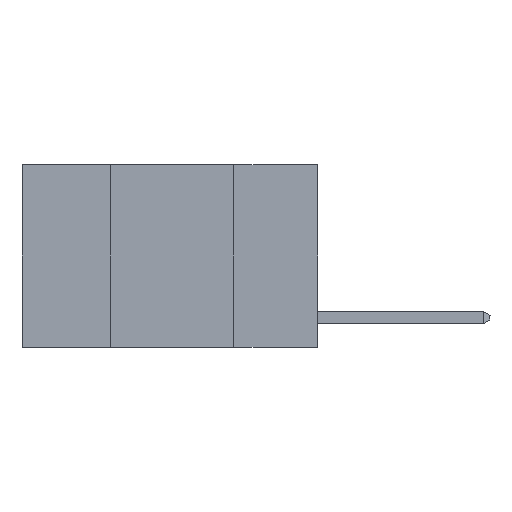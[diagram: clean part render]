
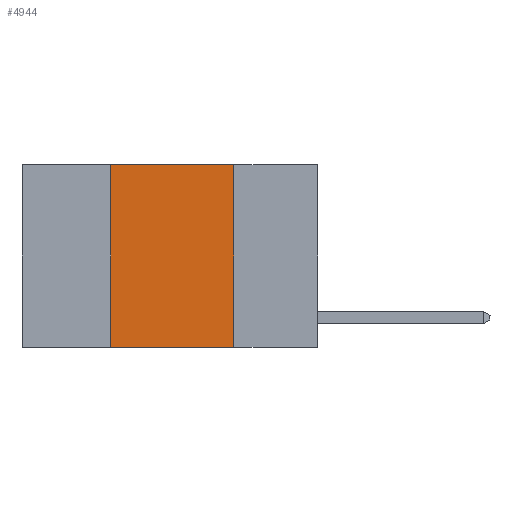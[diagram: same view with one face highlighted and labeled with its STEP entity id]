
A CAD part, left-side view. The second image highlights one B-rep face of the part: STEP entity #4944.
In plain terms, the highlighted planar face has unit normal (-1, 0, 0).
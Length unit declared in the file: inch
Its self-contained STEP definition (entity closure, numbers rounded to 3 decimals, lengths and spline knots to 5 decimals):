
#34 = DIRECTION ( 'NONE',  ( 0., 0., -1. ) ) ;
#340 = AXIS2_PLACEMENT_3D ( 'NONE', #11932, #2042, #34 ) ;
#737 = CARTESIAN_POINT ( 'NONE',  ( 0., 0.17, 0. ) ) ;
#909 = FACE_OUTER_BOUND ( 'NONE', #9807, .T. ) ;
#1210 = LINE ( 'NONE', #10998, #13427 ) ;
#2042 = DIRECTION ( 'NONE',  ( 1., 0., 0. ) ) ;
#3083 = VECTOR ( 'NONE', #8857, 39.37008 ) ;
#3143 = PLANE ( 'NONE',  #340 ) ;
#3480 = CARTESIAN_POINT ( 'NONE',  ( 0., 0.42, -0.37 ) ) ;
#3858 = LINE ( 'NONE', #4970, #11055 ) ;
#3927 = VERTEX_POINT ( 'NONE', #3480 ) ;
#3985 = DIRECTION ( 'NONE',  ( 0., -1., 0. ) ) ;
#4092 = VERTEX_POINT ( 'NONE', #737 ) ;
#4738 = EDGE_CURVE ( 'NONE', #4092, #13900, #12175, .T. ) ;
#4944 = ADVANCED_FACE ( 'NONE', ( #909 ), #3143, .F. ) ;
#4970 = CARTESIAN_POINT ( 'NONE',  ( 0., 0.42, 0. ) ) ;
#5495 = CARTESIAN_POINT ( 'NONE',  ( 0., 0.42, 0. ) ) ;
#5917 = VERTEX_POINT ( 'NONE', #5495 ) ;
#6633 = EDGE_CURVE ( 'NONE', #3927, #13900, #9477, .T. ) ;
#7908 = CARTESIAN_POINT ( 'NONE',  ( 0., 0.17, 0. ) ) ;
#7926 = EDGE_CURVE ( 'NONE', #3927, #5917, #3858, .T. ) ;
#8580 = ORIENTED_EDGE ( 'NONE', *, *, #13754, .F. ) ;
#8857 = DIRECTION ( 'NONE',  ( 0., 0., -1. ) ) ;
#9425 = DIRECTION ( 'NONE',  ( 0., 0., 1. ) ) ;
#9477 = LINE ( 'NONE', #13903, #13833 ) ;
#9784 = ORIENTED_EDGE ( 'NONE', *, *, #6633, .T. ) ;
#9807 = EDGE_LOOP ( 'NONE', ( #13290, #8580, #10019, #9784 ) ) ;
#10019 = ORIENTED_EDGE ( 'NONE', *, *, #7926, .F. ) ;
#10998 = CARTESIAN_POINT ( 'NONE',  ( 0., 0.6, 0. ) ) ;
#11055 = VECTOR ( 'NONE', #9425, 39.37008 ) ;
#11483 = DIRECTION ( 'NONE',  ( 0., -1., 0. ) ) ;
#11932 = CARTESIAN_POINT ( 'NONE',  ( 0., 0.6, 0. ) ) ;
#12061 = CARTESIAN_POINT ( 'NONE',  ( 0., 0.17, -0.37 ) ) ;
#12175 = LINE ( 'NONE', #7908, #3083 ) ;
#13290 = ORIENTED_EDGE ( 'NONE', *, *, #4738, .F. ) ;
#13427 = VECTOR ( 'NONE', #11483, 39.37008 ) ;
#13754 = EDGE_CURVE ( 'NONE', #5917, #4092, #1210, .T. ) ;
#13833 = VECTOR ( 'NONE', #3985, 39.37008 ) ;
#13900 = VERTEX_POINT ( 'NONE', #12061 ) ;
#13903 = CARTESIAN_POINT ( 'NONE',  ( 0., 0.6, -0.37 ) ) ;
